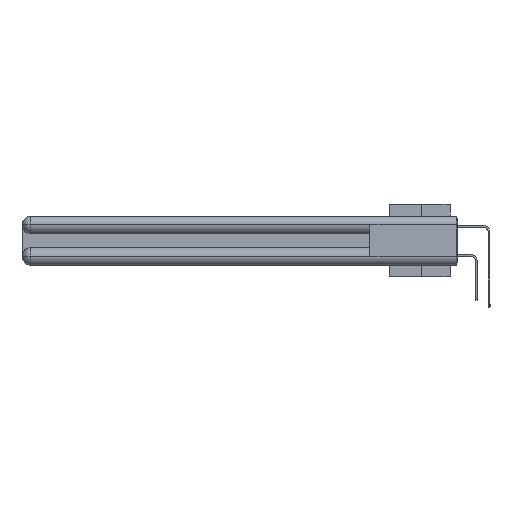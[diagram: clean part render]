
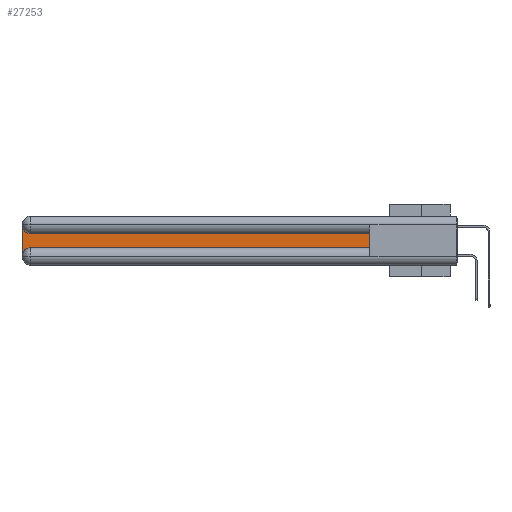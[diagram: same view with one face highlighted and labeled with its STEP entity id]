
A CAD part, left-side view. The second image highlights one B-rep face of the part: STEP entity #27253.
In plain terms, the highlighted planar face has unit normal (-1, 0, 0).
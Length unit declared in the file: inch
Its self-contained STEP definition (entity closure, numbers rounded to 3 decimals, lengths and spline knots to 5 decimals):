
#770 = DIRECTION ( 'NONE',  ( 1., 0., 0. ) ) ;
#2271 = VERTEX_POINT ( 'NONE', #8527 ) ;
#2711 = DIRECTION ( 'NONE',  ( 0., 0., 1. ) ) ;
#2833 = ORIENTED_EDGE ( 'NONE', *, *, #37177, .T. ) ;
#3260 = EDGE_CURVE ( 'NONE', #34037, #24144, #9510, .T. ) ;
#3726 = CARTESIAN_POINT ( 'NONE',  ( 0.075, 0.6, -0.2175 ) ) ;
#3815 = CARTESIAN_POINT ( 'NONE',  ( 0.075, 3., -0.2775 ) ) ;
#5686 = LINE ( 'NONE', #26308, #25442 ) ;
#6066 = DIRECTION ( 'NONE',  ( 1., 0., 0. ) ) ;
#6246 = VECTOR ( 'NONE', #15817, 39.37008 ) ;
#6319 = DIRECTION ( 'NONE',  ( 0., 0., -1. ) ) ;
#7232 = CARTESIAN_POINT ( 'NONE',  ( 0.075, 3., -0.2175 ) ) ;
#7327 = ORIENTED_EDGE ( 'NONE', *, *, #38094, .T. ) ;
#7837 = CARTESIAN_POINT ( 'NONE',  ( 0.075, 3., -0.1225 ) ) ;
#8420 = DIRECTION ( 'NONE',  ( 1., 0., 0. ) ) ;
#8527 = CARTESIAN_POINT ( 'NONE',  ( 0.075, 0.6, -0.1225 ) ) ;
#9510 = CIRCLE ( 'NONE', #19703, 0.06 ) ;
#9773 = ORIENTED_EDGE ( 'NONE', *, *, #13913, .T. ) ;
#10017 = EDGE_CURVE ( 'NONE', #24144, #34818, #30905, .T. ) ;
#10376 = CARTESIAN_POINT ( 'NONE',  ( 0.075, 2.94, -0.1225 ) ) ;
#12524 = ORIENTED_EDGE ( 'NONE', *, *, #25741, .T. ) ;
#13913 = EDGE_CURVE ( 'NONE', #2271, #20222, #18283, .T. ) ;
#15222 = AXIS2_PLACEMENT_3D ( 'NONE', #7837, #8420, #38560 ) ;
#15817 = DIRECTION ( 'NONE',  ( 0., -1., 0. ) ) ;
#16316 = ORIENTED_EDGE ( 'NONE', *, *, #3260, .T. ) ;
#17499 = DIRECTION ( 'NONE',  ( 0., 1., 0. ) ) ;
#17627 = CARTESIAN_POINT ( 'NONE',  ( 0.075, 0.6, -0.2175 ) ) ;
#18103 = CARTESIAN_POINT ( 'NONE',  ( 0.075, 3., -0.0625 ) ) ;
#18283 = LINE ( 'NONE', #33168, #24437 ) ;
#19703 = AXIS2_PLACEMENT_3D ( 'NONE', #33239, #6066, #32847 ) ;
#20222 = VERTEX_POINT ( 'NONE', #10376 ) ;
#24144 = VERTEX_POINT ( 'NONE', #34653 ) ;
#24437 = VECTOR ( 'NONE', #17499, 39.37008 ) ;
#24770 = CARTESIAN_POINT ( 'NONE',  ( 0.075, 2.94, -0.0625 ) ) ;
#25345 = VECTOR ( 'NONE', #34414, 39.37008 ) ;
#25442 = VECTOR ( 'NONE', #2711, 39.37008 ) ;
#25741 = EDGE_CURVE ( 'NONE', #26510, #34037, #27480, .T. ) ;
#26308 = CARTESIAN_POINT ( 'NONE',  ( 0.075, 0.6, -0.2175 ) ) ;
#26510 = VERTEX_POINT ( 'NONE', #18103 ) ;
#26666 = PLANE ( 'NONE',  #15222 ) ;
#27253 = ADVANCED_FACE ( 'NONE', ( #35607 ), #26666, .F. ) ;
#27480 = LINE ( 'NONE', #7232, #25345 ) ;
#28018 = CIRCLE ( 'NONE', #31811, 0.06 ) ;
#28263 = EDGE_LOOP ( 'NONE', ( #9773, #7327, #12524, #16316, #38800, #2833 ) ) ;
#30905 = LINE ( 'NONE', #3726, #6246 ) ;
#31811 = AXIS2_PLACEMENT_3D ( 'NONE', #24770, #770, #6319 ) ;
#32847 = DIRECTION ( 'NONE',  ( 0., 0., -1. ) ) ;
#33168 = CARTESIAN_POINT ( 'NONE',  ( 0.075, 0.6, -0.1225 ) ) ;
#33239 = CARTESIAN_POINT ( 'NONE',  ( 0.075, 2.94, -0.2775 ) ) ;
#34037 = VERTEX_POINT ( 'NONE', #3815 ) ;
#34414 = DIRECTION ( 'NONE',  ( 0., 0., -1. ) ) ;
#34653 = CARTESIAN_POINT ( 'NONE',  ( 0.075, 2.94, -0.2175 ) ) ;
#34818 = VERTEX_POINT ( 'NONE', #17627 ) ;
#35607 = FACE_OUTER_BOUND ( 'NONE', #28263, .T. ) ;
#37177 = EDGE_CURVE ( 'NONE', #34818, #2271, #5686, .T. ) ;
#38094 = EDGE_CURVE ( 'NONE', #20222, #26510, #28018, .T. ) ;
#38560 = DIRECTION ( 'NONE',  ( 0., 0., -1. ) ) ;
#38800 = ORIENTED_EDGE ( 'NONE', *, *, #10017, .T. ) ;
